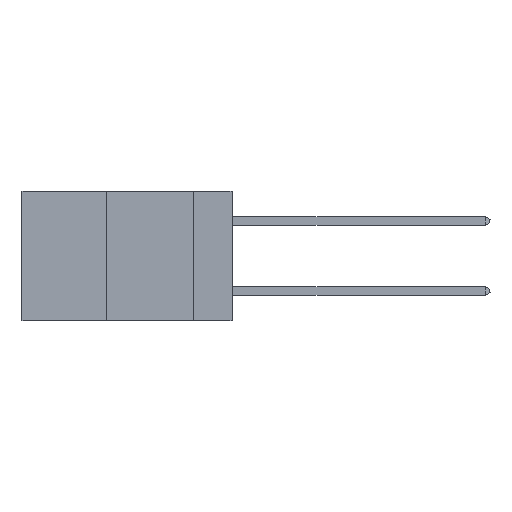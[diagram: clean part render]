
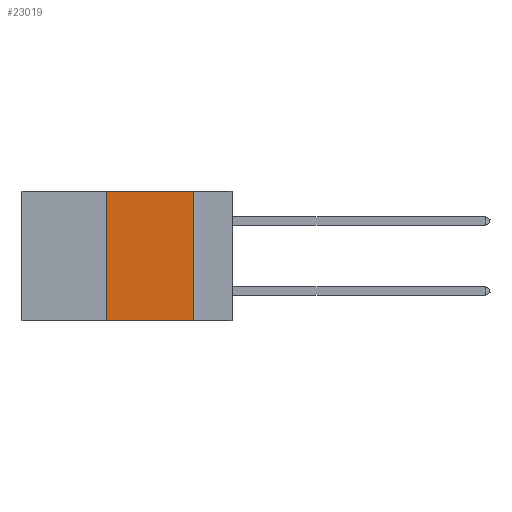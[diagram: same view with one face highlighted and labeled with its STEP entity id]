
A CAD part, left-side view. The second image highlights one B-rep face of the part: STEP entity #23019.
In plain terms, the highlighted planar face has unit normal (-1, 0, 0).
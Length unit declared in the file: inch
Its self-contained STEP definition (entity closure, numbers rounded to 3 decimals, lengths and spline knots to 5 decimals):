
#913 = CARTESIAN_POINT ( 'NONE',  ( 0., 0.36, 0. ) ) ;
#4233 = LINE ( 'NONE', #28600, #30739 ) ;
#5551 = VECTOR ( 'NONE', #28952, 39.37008 ) ;
#5949 = VERTEX_POINT ( 'NONE', #23966 ) ;
#6065 = LINE ( 'NONE', #913, #33358 ) ;
#7008 = PLANE ( 'NONE',  #23274 ) ;
#9347 = VERTEX_POINT ( 'NONE', #21765 ) ;
#10295 = VECTOR ( 'NONE', #33362, 39.37008 ) ;
#12416 = VERTEX_POINT ( 'NONE', #28130 ) ;
#12455 = DIRECTION ( 'NONE',  ( 0., 0., -1. ) ) ;
#12534 = EDGE_CURVE ( 'NONE', #9347, #5949, #4233, .T. ) ;
#13661 = EDGE_LOOP ( 'NONE', ( #23699, #23739, #24866, #25326 ) ) ;
#15018 = CARTESIAN_POINT ( 'NONE',  ( 0., 0.6, -0.37 ) ) ;
#15747 = EDGE_CURVE ( 'NONE', #12416, #9347, #6065, .T. ) ;
#19671 = DIRECTION ( 'NONE',  ( 0., 0., 1. ) ) ;
#21765 = CARTESIAN_POINT ( 'NONE',  ( 0., 0.36, 0. ) ) ;
#23016 = EDGE_CURVE ( 'NONE', #12416, #33690, #31343, .T. ) ;
#23019 = ADVANCED_FACE ( 'NONE', ( #24381 ), #7008, .F. ) ;
#23274 = AXIS2_PLACEMENT_3D ( 'NONE', #25589, #28253, #12455 ) ;
#23699 = ORIENTED_EDGE ( 'NONE', *, *, #31332, .F. ) ;
#23739 = ORIENTED_EDGE ( 'NONE', *, *, #12534, .F. ) ;
#23966 = CARTESIAN_POINT ( 'NONE',  ( 0., 0.11, 0. ) ) ;
#24381 = FACE_OUTER_BOUND ( 'NONE', #13661, .T. ) ;
#24866 = ORIENTED_EDGE ( 'NONE', *, *, #15747, .F. ) ;
#25326 = ORIENTED_EDGE ( 'NONE', *, *, #23016, .T. ) ;
#25589 = CARTESIAN_POINT ( 'NONE',  ( 0., 0.6, 0. ) ) ;
#26301 = CARTESIAN_POINT ( 'NONE',  ( 0., 0.11, 0. ) ) ;
#27014 = CARTESIAN_POINT ( 'NONE',  ( 0., 0.11, -0.37 ) ) ;
#28130 = CARTESIAN_POINT ( 'NONE',  ( 0., 0.36, -0.37 ) ) ;
#28253 = DIRECTION ( 'NONE',  ( 1., 0., 0. ) ) ;
#28600 = CARTESIAN_POINT ( 'NONE',  ( 0., 0.6, 0. ) ) ;
#28714 = DIRECTION ( 'NONE',  ( 0., -1., 0. ) ) ;
#28952 = DIRECTION ( 'NONE',  ( 0., 0., -1. ) ) ;
#30739 = VECTOR ( 'NONE', #28714, 39.37008 ) ;
#31332 = EDGE_CURVE ( 'NONE', #5949, #33690, #33672, .T. ) ;
#31343 = LINE ( 'NONE', #15018, #10295 ) ;
#33358 = VECTOR ( 'NONE', #19671, 39.37008 ) ;
#33362 = DIRECTION ( 'NONE',  ( 0., -1., 0. ) ) ;
#33672 = LINE ( 'NONE', #26301, #5551 ) ;
#33690 = VERTEX_POINT ( 'NONE', #27014 ) ;
